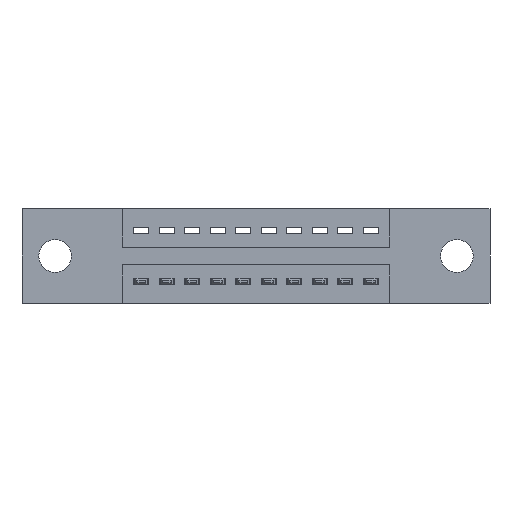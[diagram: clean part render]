
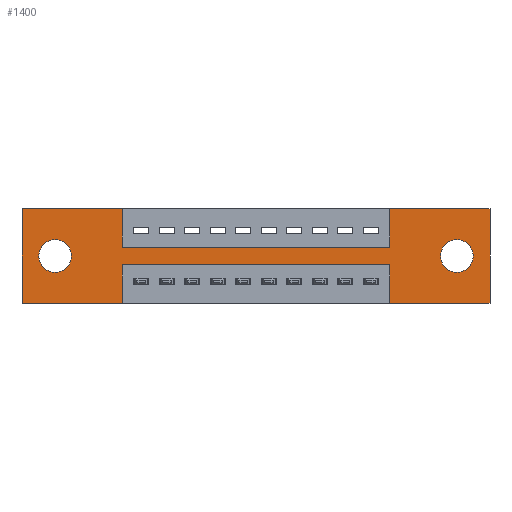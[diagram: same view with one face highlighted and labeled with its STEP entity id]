
A CAD part, front view. The second image highlights one B-rep face of the part: STEP entity #1400.
In plain terms, the highlighted planar face has unit normal (0, -1, 0).
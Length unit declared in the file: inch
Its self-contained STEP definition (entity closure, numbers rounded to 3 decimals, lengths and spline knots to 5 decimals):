
#67 = CARTESIAN_POINT ( 'NONE',  ( 1.705, 0., -0.249 ) ) ;
#68 = EDGE_CURVE ( 'NONE', #240, #9036, #526, .T. ) ;
#213 = EDGE_CURVE ( 'NONE', #9776, #5904, #5804, .T. ) ;
#224 = VECTOR ( 'NONE', #239, 39.37008 ) ;
#239 = DIRECTION ( 'NONE',  ( 0., 0., -1. ) ) ;
#240 = VERTEX_POINT ( 'NONE', #2003 ) ;
#365 = DIRECTION ( 'NONE',  ( -1., 0., 0. ) ) ;
#466 = EDGE_CURVE ( 'NONE', #9259, #240, #5253, .T. ) ;
#526 = LINE ( 'NONE', #9908, #224 ) ;
#698 = CARTESIAN_POINT ( 'NONE',  ( 1.4425, 0., -0.37 ) ) ;
#792 = EDGE_CURVE ( 'NONE', #8802, #10550, #4216, .T. ) ;
#822 = ORIENTED_EDGE ( 'NONE', *, *, #3563, .F. ) ;
#854 = VECTOR ( 'NONE', #7416, 39.37008 ) ;
#1069 = ORIENTED_EDGE ( 'NONE', *, *, #7275, .F. ) ;
#1070 = CIRCLE ( 'NONE', #7942, 0.064 ) ;
#1079 = ORIENTED_EDGE ( 'NONE', *, *, #10581, .T. ) ;
#1116 = ORIENTED_EDGE ( 'NONE', *, *, #213, .F. ) ;
#1191 = EDGE_CURVE ( 'NONE', #3906, #3589, #9234, .T. ) ;
#1277 = CARTESIAN_POINT ( 'NONE',  ( 1.835, 0., -0.37 ) ) ;
#1326 = VECTOR ( 'NONE', #11126, 39.37008 ) ;
#1337 = LINE ( 'NONE', #8334, #10868 ) ;
#1358 = CIRCLE ( 'NONE', #6753, 0.064 ) ;
#1400 = ADVANCED_FACE ( 'NONE', ( #10919, #1669, #6222 ), #10040, .T. ) ;
#1548 = ORIENTED_EDGE ( 'NONE', *, *, #4602, .F. ) ;
#1592 = DIRECTION ( 'NONE',  ( 0., 1., 0. ) ) ;
#1641 = ORIENTED_EDGE ( 'NONE', *, *, #466, .F. ) ;
#1643 = DIRECTION ( 'NONE',  ( 0., 0., 1. ) ) ;
#1669 = FACE_BOUND ( 'NONE', #11523, .T. ) ;
#1731 = LINE ( 'NONE', #3181, #9150 ) ;
#1763 = ORIENTED_EDGE ( 'NONE', *, *, #68, .F. ) ;
#1916 = CARTESIAN_POINT ( 'NONE',  ( 0.3925, 0., 0. ) ) ;
#1924 = CARTESIAN_POINT ( 'NONE',  ( 0.3925, 0., -0.37 ) ) ;
#1966 = DIRECTION ( 'NONE',  ( 0., 0., -1. ) ) ;
#1980 = ORIENTED_EDGE ( 'NONE', *, *, #11548, .F. ) ;
#2003 = CARTESIAN_POINT ( 'NONE',  ( 1.835, 0., 0. ) ) ;
#2138 = EDGE_CURVE ( 'NONE', #2649, #8176, #11434, .T. ) ;
#2217 = ORIENTED_EDGE ( 'NONE', *, *, #6361, .F. ) ;
#2289 = ORIENTED_EDGE ( 'NONE', *, *, #6564, .T. ) ;
#2345 = ORIENTED_EDGE ( 'NONE', *, *, #2138, .T. ) ;
#2396 = CARTESIAN_POINT ( 'NONE',  ( 0., 0., 0. ) ) ;
#2461 = DIRECTION ( 'NONE',  ( -1., 0., 0. ) ) ;
#2519 = AXIS2_PLACEMENT_3D ( 'NONE', #9224, #9206, #9198 ) ;
#2535 = CARTESIAN_POINT ( 'NONE',  ( 0., 0., 0. ) ) ;
#2610 = DIRECTION ( 'NONE',  ( 0., 1., 0. ) ) ;
#2649 = VERTEX_POINT ( 'NONE', #6050 ) ;
#2683 = DIRECTION ( 'NONE',  ( 1., 0., 0. ) ) ;
#2710 = EDGE_LOOP ( 'NONE', ( #2345, #6840 ) ) ;
#3128 = CARTESIAN_POINT ( 'NONE',  ( 0., 0., 0. ) ) ;
#3139 = DIRECTION ( 'NONE',  ( 1., 0., 0. ) ) ;
#3149 = EDGE_CURVE ( 'NONE', #8583, #5357, #5594, .T. ) ;
#3166 = AXIS2_PLACEMENT_3D ( 'NONE', #11493, #9958, #9914 ) ;
#3181 = CARTESIAN_POINT ( 'NONE',  ( 0.3925, 0., -0.15 ) ) ;
#3201 = CARTESIAN_POINT ( 'NONE',  ( 0., 0., -0.37 ) ) ;
#3315 = AXIS2_PLACEMENT_3D ( 'NONE', #7015, #1592, #7912 ) ;
#3476 = CARTESIAN_POINT ( 'NONE',  ( 0.13, 0., -0.185 ) ) ;
#3514 = CARTESIAN_POINT ( 'NONE',  ( 1.4425, 0., -0.22 ) ) ;
#3563 = EDGE_CURVE ( 'NONE', #5357, #9776, #1337, .T. ) ;
#3589 = VERTEX_POINT ( 'NONE', #3514 ) ;
#3906 = VERTEX_POINT ( 'NONE', #698 ) ;
#3972 = EDGE_CURVE ( 'NONE', #5904, #8802, #8479, .T. ) ;
#4216 = LINE ( 'NONE', #5261, #8703 ) ;
#4295 = CARTESIAN_POINT ( 'NONE',  ( 0.3925, 0., -0.15 ) ) ;
#4383 = DIRECTION ( 'NONE',  ( 0., 0., 1. ) ) ;
#4602 = EDGE_CURVE ( 'NONE', #10550, #10132, #1731, .T. ) ;
#4681 = CARTESIAN_POINT ( 'NONE',  ( 1.4425, 0., -0.15 ) ) ;
#4813 = ORIENTED_EDGE ( 'NONE', *, *, #1191, .F. ) ;
#5253 = LINE ( 'NONE', #5646, #7360 ) ;
#5261 = CARTESIAN_POINT ( 'NONE',  ( 0.3925, 0., 0. ) ) ;
#5263 = DIRECTION ( 'NONE',  ( 0., 0., -1. ) ) ;
#5293 = VECTOR ( 'NONE', #365, 39.37008 ) ;
#5320 = VECTOR ( 'NONE', #1966, 39.37008 ) ;
#5357 = VERTEX_POINT ( 'NONE', #8674 ) ;
#5512 = VECTOR ( 'NONE', #10301, 39.37008 ) ;
#5535 = ORIENTED_EDGE ( 'NONE', *, *, #3149, .F. ) ;
#5594 = LINE ( 'NONE', #1924, #5320 ) ;
#5646 = CARTESIAN_POINT ( 'NONE',  ( 0., 0., 0. ) ) ;
#5804 = LINE ( 'NONE', #3128, #5512 ) ;
#5904 = VERTEX_POINT ( 'NONE', #2396 ) ;
#6050 = CARTESIAN_POINT ( 'NONE',  ( 1.705, 0., -0.121 ) ) ;
#6222 = FACE_OUTER_BOUND ( 'NONE', #8654, .T. ) ;
#6361 = EDGE_CURVE ( 'NONE', #9036, #3906, #7950, .T. ) ;
#6521 = CARTESIAN_POINT ( 'NONE',  ( 1.4425, 0., 0. ) ) ;
#6564 = EDGE_CURVE ( 'NONE', #9270, #10704, #8341, .T. ) ;
#6753 = AXIS2_PLACEMENT_3D ( 'NONE', #3476, #9727, #4383 ) ;
#6840 = ORIENTED_EDGE ( 'NONE', *, *, #10598, .T. ) ;
#7015 = CARTESIAN_POINT ( 'NONE',  ( 0.13, 0., -0.185 ) ) ;
#7275 = EDGE_CURVE ( 'NONE', #3589, #8583, #7930, .T. ) ;
#7360 = VECTOR ( 'NONE', #2683, 39.37008 ) ;
#7416 = DIRECTION ( 'NONE',  ( 0., 0., 1. ) ) ;
#7511 = CARTESIAN_POINT ( 'NONE',  ( 1.4425, 0., -0.37 ) ) ;
#7648 = VECTOR ( 'NONE', #2461, 39.37008 ) ;
#7912 = DIRECTION ( 'NONE',  ( 0., 0., 1. ) ) ;
#7930 = LINE ( 'NONE', #11318, #7648 ) ;
#7942 = AXIS2_PLACEMENT_3D ( 'NONE', #8008, #2610, #8860 ) ;
#7950 = LINE ( 'NONE', #8498, #5293 ) ;
#7962 = CARTESIAN_POINT ( 'NONE',  ( 0.13, 0., -0.121 ) ) ;
#8008 = CARTESIAN_POINT ( 'NONE',  ( 1.705, 0., -0.185 ) ) ;
#8115 = CARTESIAN_POINT ( 'NONE',  ( 0.13, 0., -0.249 ) ) ;
#8124 = DIRECTION ( 'NONE',  ( -1., 0., 0. ) ) ;
#8176 = VERTEX_POINT ( 'NONE', #67 ) ;
#8334 = CARTESIAN_POINT ( 'NONE',  ( 0., 0., -0.37 ) ) ;
#8341 = CIRCLE ( 'NONE', #3315, 0.064 ) ;
#8479 = LINE ( 'NONE', #2535, #1326 ) ;
#8498 = CARTESIAN_POINT ( 'NONE',  ( 0., 0., -0.37 ) ) ;
#8583 = VERTEX_POINT ( 'NONE', #8795 ) ;
#8654 = EDGE_LOOP ( 'NONE', ( #5535, #1069, #4813, #2217, #1763, #1641, #1980, #1548, #9507, #9214, #1116, #822 ) ) ;
#8674 = CARTESIAN_POINT ( 'NONE',  ( 0.3925, 0., -0.37 ) ) ;
#8703 = VECTOR ( 'NONE', #5263, 39.37008 ) ;
#8795 = CARTESIAN_POINT ( 'NONE',  ( 0.3925, 0., -0.22 ) ) ;
#8802 = VERTEX_POINT ( 'NONE', #1916 ) ;
#8860 = DIRECTION ( 'NONE',  ( 0., 0., -1. ) ) ;
#8946 = VECTOR ( 'NONE', #1643, 39.37008 ) ;
#9036 = VERTEX_POINT ( 'NONE', #1277 ) ;
#9150 = VECTOR ( 'NONE', #3139, 39.37008 ) ;
#9198 = DIRECTION ( 'NONE',  ( 0., 0., -1. ) ) ;
#9206 = DIRECTION ( 'NONE',  ( 0., 1., 0. ) ) ;
#9214 = ORIENTED_EDGE ( 'NONE', *, *, #3972, .F. ) ;
#9224 = CARTESIAN_POINT ( 'NONE',  ( 1.705, 0., -0.185 ) ) ;
#9234 = LINE ( 'NONE', #7511, #8946 ) ;
#9259 = VERTEX_POINT ( 'NONE', #9608 ) ;
#9270 = VERTEX_POINT ( 'NONE', #7962 ) ;
#9507 = ORIENTED_EDGE ( 'NONE', *, *, #792, .F. ) ;
#9608 = CARTESIAN_POINT ( 'NONE',  ( 1.4425, 0., 0. ) ) ;
#9727 = DIRECTION ( 'NONE',  ( 0., 1., 0. ) ) ;
#9776 = VERTEX_POINT ( 'NONE', #3201 ) ;
#9908 = CARTESIAN_POINT ( 'NONE',  ( 1.835, 0., 0. ) ) ;
#9914 = DIRECTION ( 'NONE',  ( 0., 0., -1. ) ) ;
#9958 = DIRECTION ( 'NONE',  ( 0., -1., 0. ) ) ;
#10040 = PLANE ( 'NONE',  #3166 ) ;
#10132 = VERTEX_POINT ( 'NONE', #4681 ) ;
#10301 = DIRECTION ( 'NONE',  ( 0., 0., 1. ) ) ;
#10406 = LINE ( 'NONE', #6521, #854 ) ;
#10550 = VERTEX_POINT ( 'NONE', #4295 ) ;
#10581 = EDGE_CURVE ( 'NONE', #10704, #9270, #1358, .T. ) ;
#10598 = EDGE_CURVE ( 'NONE', #8176, #2649, #1070, .T. ) ;
#10704 = VERTEX_POINT ( 'NONE', #8115 ) ;
#10868 = VECTOR ( 'NONE', #8124, 39.37008 ) ;
#10919 = FACE_BOUND ( 'NONE', #2710, .T. ) ;
#11126 = DIRECTION ( 'NONE',  ( 1., 0., 0. ) ) ;
#11318 = CARTESIAN_POINT ( 'NONE',  ( 0.3925, 0., -0.22 ) ) ;
#11434 = CIRCLE ( 'NONE', #2519, 0.064 ) ;
#11493 = CARTESIAN_POINT ( 'NONE',  ( 0., 0., -0.37 ) ) ;
#11523 = EDGE_LOOP ( 'NONE', ( #2289, #1079 ) ) ;
#11548 = EDGE_CURVE ( 'NONE', #10132, #9259, #10406, .T. ) ;
